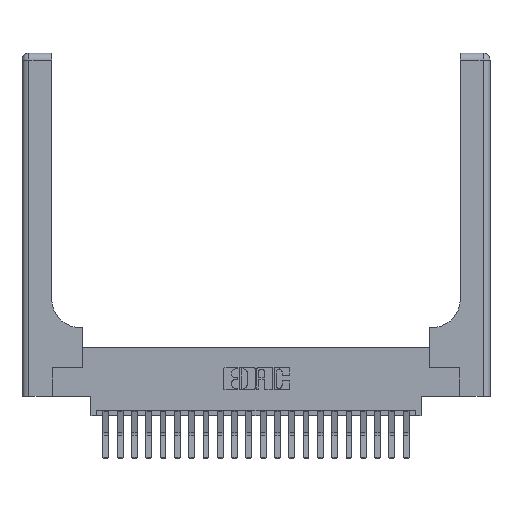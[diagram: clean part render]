
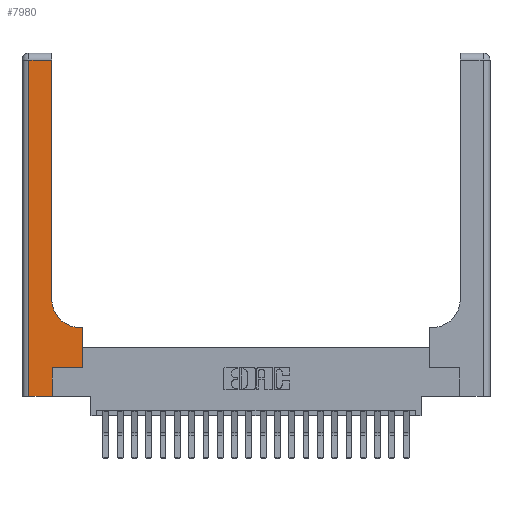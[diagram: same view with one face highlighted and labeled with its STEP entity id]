
A CAD part, top view. The second image highlights one B-rep face of the part: STEP entity #7980.
In plain terms, the highlighted planar face has unit normal (0, 0, 1).
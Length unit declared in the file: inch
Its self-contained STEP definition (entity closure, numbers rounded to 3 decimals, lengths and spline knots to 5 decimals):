
#70 = VERTEX_POINT ( 'NONE', #10797 ) ;
#716 = ORIENTED_EDGE ( 'NONE', *, *, #10520, .T. ) ;
#779 = DIRECTION ( 'NONE',  ( 0., -1., 0. ) ) ;
#830 = CARTESIAN_POINT ( 'NONE',  ( 0.265, 0.25, 0.37 ) ) ;
#1044 = AXIS2_PLACEMENT_3D ( 'NONE', #12435, #1925, #14159 ) ;
#1481 = DIRECTION ( 'NONE',  ( 0., 0., -1. ) ) ;
#1536 = VECTOR ( 'NONE', #779, 39.37008 ) ;
#1610 = VERTEX_POINT ( 'NONE', #19160 ) ;
#1697 = CARTESIAN_POINT ( 'NONE',  ( 0.26, 0.6, 0.37 ) ) ;
#1925 = DIRECTION ( 'NONE',  ( 0., 0., -1. ) ) ;
#2077 = LINE ( 'NONE', #12966, #1536 ) ;
#2959 = CARTESIAN_POINT ( 'NONE',  ( 0.265, 0., 0.37 ) ) ;
#3361 = ORIENTED_EDGE ( 'NONE', *, *, #16993, .T. ) ;
#3432 = VECTOR ( 'NONE', #17444, 39.37008 ) ;
#3526 = LINE ( 'NONE', #4560, #4056 ) ;
#3847 = LINE ( 'NONE', #1697, #20662 ) ;
#4056 = VECTOR ( 'NONE', #16730, 39.37008 ) ;
#4381 = DIRECTION ( 'NONE',  ( -1., 0., 0. ) ) ;
#4505 = VECTOR ( 'NONE', #11018, 39.37008 ) ;
#4519 = DIRECTION ( 'NONE',  ( 0., 1., 0. ) ) ;
#4560 = CARTESIAN_POINT ( 'NONE',  ( 0.528, 0.25, 0.37 ) ) ;
#4713 = ORIENTED_EDGE ( 'NONE', *, *, #20649, .T. ) ;
#4826 = EDGE_CURVE ( 'NONE', #21380, #22415, #2077, .T. ) ;
#4918 = EDGE_CURVE ( 'NONE', #18072, #8861, #13855, .T. ) ;
#5293 = CARTESIAN_POINT ( 'NONE',  ( 0.26, 3., 0.37 ) ) ;
#5722 = CARTESIAN_POINT ( 'NONE',  ( 0., 0., 0.37 ) ) ;
#6069 = ORIENTED_EDGE ( 'NONE', *, *, #11142, .T. ) ;
#6888 = CARTESIAN_POINT ( 'NONE',  ( 0.26, 2.94, 0.37 ) ) ;
#7064 = ORIENTED_EDGE ( 'NONE', *, *, #14196, .T. ) ;
#7439 = CARTESIAN_POINT ( 'NONE',  ( 0.528, 0.25, 0.37 ) ) ;
#7980 = ADVANCED_FACE ( 'NONE', ( #21746 ), #8929, .F. ) ;
#8694 = VECTOR ( 'NONE', #4519, 39.37008 ) ;
#8712 = VERTEX_POINT ( 'NONE', #7439 ) ;
#8861 = VERTEX_POINT ( 'NONE', #830 ) ;
#8929 = PLANE ( 'NONE',  #1044 ) ;
#9540 = ORIENTED_EDGE ( 'NONE', *, *, #4918, .T. ) ;
#9554 = VECTOR ( 'NONE', #4381, 39.37008 ) ;
#9559 = ORIENTED_EDGE ( 'NONE', *, *, #20358, .T. ) ;
#9716 = CARTESIAN_POINT ( 'NONE',  ( 0., 2.94, 0.37 ) ) ;
#10006 = CIRCLE ( 'NONE', #12437, 0.25 ) ;
#10460 = DIRECTION ( 'NONE',  ( -1., 0., 0. ) ) ;
#10520 = EDGE_CURVE ( 'NONE', #8712, #70, #3526, .T. ) ;
#10640 = LINE ( 'NONE', #9716, #9554 ) ;
#10797 = CARTESIAN_POINT ( 'NONE',  ( 0.528, 0.6, 0.37 ) ) ;
#11018 = DIRECTION ( 'NONE',  ( 1., 0., 0. ) ) ;
#11142 = EDGE_CURVE ( 'NONE', #18221, #21380, #10640, .T. ) ;
#11182 = ORIENTED_EDGE ( 'NONE', *, *, #4826, .T. ) ;
#11435 = CARTESIAN_POINT ( 'NONE',  ( 0.265, 0.25, 0.37 ) ) ;
#11738 = ORIENTED_EDGE ( 'NONE', *, *, #13433, .T. ) ;
#12006 = CARTESIAN_POINT ( 'NONE',  ( 0.51, 0.85, 0.37 ) ) ;
#12435 = CARTESIAN_POINT ( 'NONE',  ( 0., 3., 0.37 ) ) ;
#12437 = AXIS2_PLACEMENT_3D ( 'NONE', #12006, #1481, #13734 ) ;
#12966 = CARTESIAN_POINT ( 'NONE',  ( 0.06, 3., 0.37 ) ) ;
#13433 = EDGE_CURVE ( 'NONE', #22415, #18072, #18379, .T. ) ;
#13734 = DIRECTION ( 'NONE',  ( 1., 0., 0. ) ) ;
#13855 = LINE ( 'NONE', #14989, #8694 ) ;
#14159 = DIRECTION ( 'NONE',  ( -1., 0., 0. ) ) ;
#14196 = EDGE_CURVE ( 'NONE', #1610, #18256, #10006, .T. ) ;
#14989 = CARTESIAN_POINT ( 'NONE',  ( 0.265, 0., 0.37 ) ) ;
#15896 = CARTESIAN_POINT ( 'NONE',  ( 0.06, 2.94, 0.37 ) ) ;
#16606 = VECTOR ( 'NONE', #21498, 39.37008 ) ;
#16730 = DIRECTION ( 'NONE',  ( 0., 1., 0. ) ) ;
#16977 = CARTESIAN_POINT ( 'NONE',  ( 0.06, 0., 0.37 ) ) ;
#16993 = EDGE_CURVE ( 'NONE', #18256, #18221, #22403, .T. ) ;
#17444 = DIRECTION ( 'NONE',  ( 0., 1., 0. ) ) ;
#17681 = LINE ( 'NONE', #11435, #16606 ) ;
#18072 = VERTEX_POINT ( 'NONE', #2959 ) ;
#18221 = VERTEX_POINT ( 'NONE', #6888 ) ;
#18256 = VERTEX_POINT ( 'NONE', #19144 ) ;
#18379 = LINE ( 'NONE', #5722, #4505 ) ;
#19144 = CARTESIAN_POINT ( 'NONE',  ( 0.26, 0.85, 0.37 ) ) ;
#19160 = CARTESIAN_POINT ( 'NONE',  ( 0.51, 0.6, 0.37 ) ) ;
#19953 = EDGE_LOOP ( 'NONE', ( #3361, #6069, #11182, #11738, #9540, #9559, #716, #4713, #7064 ) ) ;
#20358 = EDGE_CURVE ( 'NONE', #8861, #8712, #17681, .T. ) ;
#20649 = EDGE_CURVE ( 'NONE', #70, #1610, #3847, .T. ) ;
#20662 = VECTOR ( 'NONE', #10460, 39.37008 ) ;
#21380 = VERTEX_POINT ( 'NONE', #15896 ) ;
#21498 = DIRECTION ( 'NONE',  ( 1., 0., 0. ) ) ;
#21746 = FACE_OUTER_BOUND ( 'NONE', #19953, .T. ) ;
#22403 = LINE ( 'NONE', #5293, #3432 ) ;
#22415 = VERTEX_POINT ( 'NONE', #16977 ) ;
